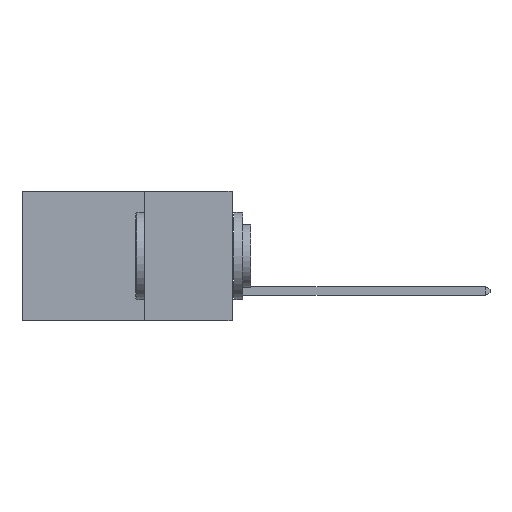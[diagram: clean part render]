
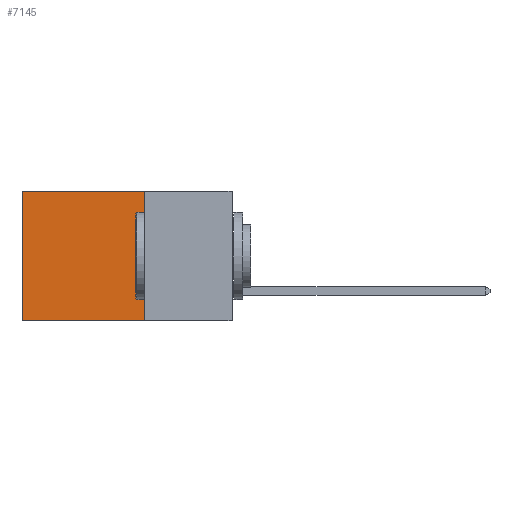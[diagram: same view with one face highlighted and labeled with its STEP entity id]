
A CAD part, left-side view. The second image highlights one B-rep face of the part: STEP entity #7145.
In plain terms, the highlighted planar face has unit normal (-1, 0, 0).
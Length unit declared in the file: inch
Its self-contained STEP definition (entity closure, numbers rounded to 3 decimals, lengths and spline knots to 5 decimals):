
#733 = VECTOR ( 'NONE', #7203, 39.37008 ) ;
#967 = PLANE ( 'NONE',  #2729 ) ;
#1867 = EDGE_CURVE ( 'NONE', #9411, #8082, #12819, .T. ) ;
#2007 = ORIENTED_EDGE ( 'NONE', *, *, #6550, .T. ) ;
#2264 = VECTOR ( 'NONE', #8949, 39.37008 ) ;
#2266 = ORIENTED_EDGE ( 'NONE', *, *, #1867, .F. ) ;
#2729 = AXIS2_PLACEMENT_3D ( 'NONE', #8008, #9004, #2970 ) ;
#2959 = VERTEX_POINT ( 'NONE', #7491 ) ;
#2970 = DIRECTION ( 'NONE',  ( 0., 0., -1. ) ) ;
#3806 = VECTOR ( 'NONE', #11041, 39.37008 ) ;
#3827 = ORIENTED_EDGE ( 'NONE', *, *, #9781, .T. ) ;
#4069 = CARTESIAN_POINT ( 'NONE',  ( 0.2875, 0.25, 0. ) ) ;
#4075 = LINE ( 'NONE', #7544, #6488 ) ;
#4937 = VERTEX_POINT ( 'NONE', #11749 ) ;
#5098 = EDGE_LOOP ( 'NONE', ( #2007, #8694, #2266, #3827 ) ) ;
#5733 = CARTESIAN_POINT ( 'NONE',  ( 0.2875, 0.25, -0.37 ) ) ;
#6119 = CARTESIAN_POINT ( 'NONE',  ( 0.2875, 0.6, 0. ) ) ;
#6488 = VECTOR ( 'NONE', #6598, 39.37008 ) ;
#6550 = EDGE_CURVE ( 'NONE', #4937, #2959, #11752, .T. ) ;
#6598 = DIRECTION ( 'NONE',  ( 0., 1., 0. ) ) ;
#6723 = CARTESIAN_POINT ( 'NONE',  ( 0.2875, 0.25, 0. ) ) ;
#7145 = ADVANCED_FACE ( 'NONE', ( #7286 ), #967, .F. ) ;
#7203 = DIRECTION ( 'NONE',  ( 0., 1., 0. ) ) ;
#7286 = FACE_OUTER_BOUND ( 'NONE', #5098, .T. ) ;
#7491 = CARTESIAN_POINT ( 'NONE',  ( 0.2875, 0.6, -0.37 ) ) ;
#7544 = CARTESIAN_POINT ( 'NONE',  ( 0.2875, 0.25, -0.37 ) ) ;
#8008 = CARTESIAN_POINT ( 'NONE',  ( 0.2875, 0.25, 0. ) ) ;
#8082 = VERTEX_POINT ( 'NONE', #5733 ) ;
#8694 = ORIENTED_EDGE ( 'NONE', *, *, #9316, .F. ) ;
#8747 = LINE ( 'NONE', #4069, #733 ) ;
#8949 = DIRECTION ( 'NONE',  ( 0., 0., -1. ) ) ;
#9004 = DIRECTION ( 'NONE',  ( 1., 0., 0. ) ) ;
#9316 = EDGE_CURVE ( 'NONE', #8082, #2959, #4075, .T. ) ;
#9411 = VERTEX_POINT ( 'NONE', #6723 ) ;
#9781 = EDGE_CURVE ( 'NONE', #9411, #4937, #8747, .T. ) ;
#11041 = DIRECTION ( 'NONE',  ( 0., 0., -1. ) ) ;
#11749 = CARTESIAN_POINT ( 'NONE',  ( 0.2875, 0.6, 0. ) ) ;
#11752 = LINE ( 'NONE', #6119, #3806 ) ;
#12788 = CARTESIAN_POINT ( 'NONE',  ( 0.2875, 0.25, 0. ) ) ;
#12819 = LINE ( 'NONE', #12788, #2264 ) ;
